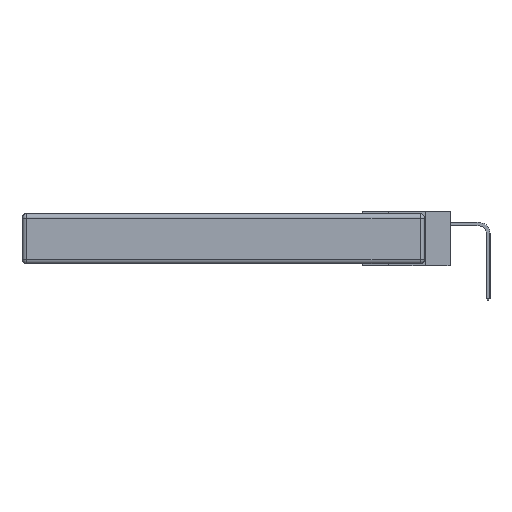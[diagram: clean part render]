
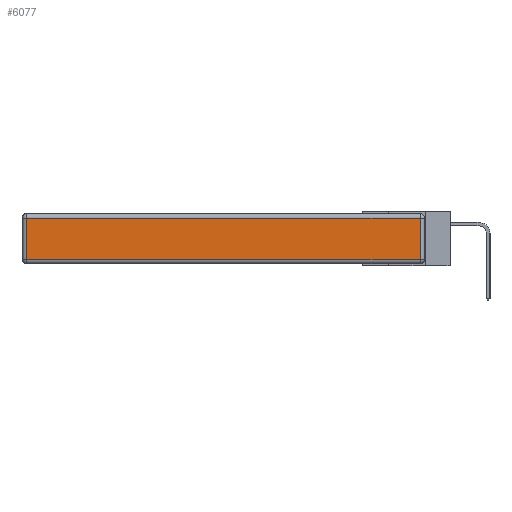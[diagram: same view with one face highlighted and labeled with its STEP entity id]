
A CAD part, left-side view. The second image highlights one B-rep face of the part: STEP entity #6077.
In plain terms, the highlighted planar face has unit normal (-1, 0, 0).
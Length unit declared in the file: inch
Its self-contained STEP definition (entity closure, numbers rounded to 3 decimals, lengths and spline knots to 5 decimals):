
#588 = LINE ( 'NONE', #4617, #5051 ) ;
#631 = CARTESIAN_POINT ( 'NONE',  ( 0., 2.72, -0.313 ) ) ;
#1258 = DIRECTION ( 'NONE',  ( 0., 0., -1. ) ) ;
#1572 = VECTOR ( 'NONE', #8519, 39.37008 ) ;
#1616 = AXIS2_PLACEMENT_3D ( 'NONE', #20110, #8844, #20985 ) ;
#4082 = EDGE_CURVE ( 'NONE', #14599, #18802, #17082, .T. ) ;
#4617 = CARTESIAN_POINT ( 'NONE',  ( 0., 0., -0.313 ) ) ;
#4657 = VECTOR ( 'NONE', #1258, 39.37008 ) ;
#5051 = VECTOR ( 'NONE', #21982, 39.37008 ) ;
#6077 = ADVANCED_FACE ( 'NONE', ( #9668 ), #18214, .T. ) ;
#6243 = ORIENTED_EDGE ( 'NONE', *, *, #8783, .T. ) ;
#6287 = EDGE_CURVE ( 'NONE', #14672, #13716, #22601, .T. ) ;
#8519 = DIRECTION ( 'NONE',  ( 0., 1., 0. ) ) ;
#8783 = EDGE_CURVE ( 'NONE', #13716, #14599, #588, .T. ) ;
#8844 = DIRECTION ( 'NONE',  ( -1., 0., 0. ) ) ;
#9538 = CARTESIAN_POINT ( 'NONE',  ( 0., 2.72, -0.343 ) ) ;
#9668 = FACE_OUTER_BOUND ( 'NONE', #18155, .T. ) ;
#11134 = ORIENTED_EDGE ( 'NONE', *, *, #4082, .T. ) ;
#12857 = ORIENTED_EDGE ( 'NONE', *, *, #14320, .T. ) ;
#13716 = VERTEX_POINT ( 'NONE', #631 ) ;
#13902 = LINE ( 'NONE', #16196, #1572 ) ;
#14320 = EDGE_CURVE ( 'NONE', #18802, #14672, #13902, .T. ) ;
#14599 = VERTEX_POINT ( 'NONE', #22075 ) ;
#14672 = VERTEX_POINT ( 'NONE', #23334 ) ;
#14705 = VECTOR ( 'NONE', #16238, 39.37008 ) ;
#15575 = CARTESIAN_POINT ( 'NONE',  ( 0., 0.03, -0.343 ) ) ;
#15983 = ORIENTED_EDGE ( 'NONE', *, *, #6287, .T. ) ;
#16196 = CARTESIAN_POINT ( 'NONE',  ( 0., 2.75, -0.03 ) ) ;
#16238 = DIRECTION ( 'NONE',  ( 0., 0., 1. ) ) ;
#17082 = LINE ( 'NONE', #15575, #14705 ) ;
#18155 = EDGE_LOOP ( 'NONE', ( #6243, #11134, #12857, #15983 ) ) ;
#18214 = PLANE ( 'NONE',  #1616 ) ;
#18802 = VERTEX_POINT ( 'NONE', #23633 ) ;
#20110 = CARTESIAN_POINT ( 'NONE',  ( 0., 0., -0.343 ) ) ;
#20985 = DIRECTION ( 'NONE',  ( 0., 0., 1. ) ) ;
#21982 = DIRECTION ( 'NONE',  ( 0., -1., 0. ) ) ;
#22075 = CARTESIAN_POINT ( 'NONE',  ( 0., 0.03, -0.313 ) ) ;
#22601 = LINE ( 'NONE', #9538, #4657 ) ;
#23334 = CARTESIAN_POINT ( 'NONE',  ( 0., 2.72, -0.03 ) ) ;
#23633 = CARTESIAN_POINT ( 'NONE',  ( 0., 0.03, -0.03 ) ) ;
